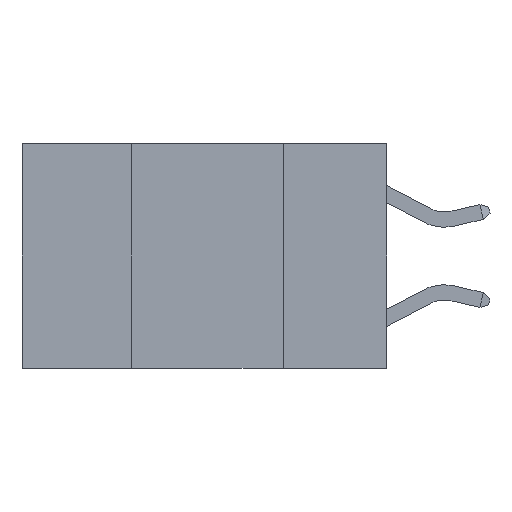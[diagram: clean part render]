
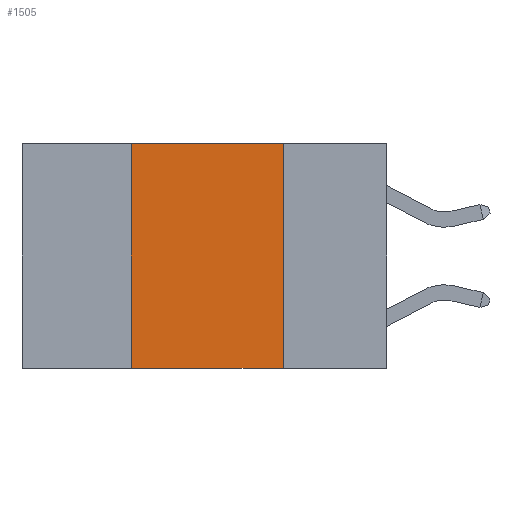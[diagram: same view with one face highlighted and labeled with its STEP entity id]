
A CAD part, left-side view. The second image highlights one B-rep face of the part: STEP entity #1505.
In plain terms, the highlighted planar face has unit normal (-1, 0, 0).
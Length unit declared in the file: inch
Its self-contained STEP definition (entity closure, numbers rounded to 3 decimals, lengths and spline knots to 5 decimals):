
#339 = CARTESIAN_POINT ( 'NONE',  ( 0., 0.17, 0. ) ) ;
#483 = DIRECTION ( 'NONE',  ( 0., 0., 1. ) ) ;
#638 = DIRECTION ( 'NONE',  ( 0., -1., 0. ) ) ;
#950 = CARTESIAN_POINT ( 'NONE',  ( 0., 0.42, 0. ) ) ;
#1000 = VERTEX_POINT ( 'NONE', #4841 ) ;
#1066 = ORIENTED_EDGE ( 'NONE', *, *, #4384, .F. ) ;
#1128 = ORIENTED_EDGE ( 'NONE', *, *, #9726, .F. ) ;
#1137 = ORIENTED_EDGE ( 'NONE', *, *, #7871, .F. ) ;
#1216 = ORIENTED_EDGE ( 'NONE', *, *, #9218, .T. ) ;
#1371 = LINE ( 'NONE', #10041, #9614 ) ;
#1448 = CARTESIAN_POINT ( 'NONE',  ( 0., 0.42, -0.37 ) ) ;
#1505 = ADVANCED_FACE ( 'NONE', ( #4054 ), #2996, .F. ) ;
#1510 = VERTEX_POINT ( 'NONE', #339 ) ;
#1856 = VERTEX_POINT ( 'NONE', #950 ) ;
#2473 = AXIS2_PLACEMENT_3D ( 'NONE', #3830, #4743, #10279 ) ;
#2729 = DIRECTION ( 'NONE',  ( 0., -1., 0. ) ) ;
#2772 = LINE ( 'NONE', #5670, #4814 ) ;
#2848 = EDGE_LOOP ( 'NONE', ( #1066, #1128, #1137, #1216 ) ) ;
#2996 = PLANE ( 'NONE',  #2473 ) ;
#3026 = LINE ( 'NONE', #10499, #7190 ) ;
#3674 = VECTOR ( 'NONE', #8176, 39.37008 ) ;
#3830 = CARTESIAN_POINT ( 'NONE',  ( 0., 0.6, 0. ) ) ;
#4054 = FACE_OUTER_BOUND ( 'NONE', #2848, .T. ) ;
#4384 = EDGE_CURVE ( 'NONE', #1510, #1000, #8034, .T. ) ;
#4743 = DIRECTION ( 'NONE',  ( 1., 0., 0. ) ) ;
#4814 = VECTOR ( 'NONE', #483, 39.37008 ) ;
#4841 = CARTESIAN_POINT ( 'NONE',  ( 0., 0.17, -0.37 ) ) ;
#5670 = CARTESIAN_POINT ( 'NONE',  ( 0., 0.42, 0. ) ) ;
#7190 = VECTOR ( 'NONE', #638, 39.37008 ) ;
#7871 = EDGE_CURVE ( 'NONE', #8722, #1856, #2772, .T. ) ;
#8034 = LINE ( 'NONE', #9678, #3674 ) ;
#8176 = DIRECTION ( 'NONE',  ( 0., 0., -1. ) ) ;
#8722 = VERTEX_POINT ( 'NONE', #1448 ) ;
#9218 = EDGE_CURVE ( 'NONE', #8722, #1000, #1371, .T. ) ;
#9614 = VECTOR ( 'NONE', #2729, 39.37008 ) ;
#9678 = CARTESIAN_POINT ( 'NONE',  ( 0., 0.17, 0. ) ) ;
#9726 = EDGE_CURVE ( 'NONE', #1856, #1510, #3026, .T. ) ;
#10041 = CARTESIAN_POINT ( 'NONE',  ( 0., 0.6, -0.37 ) ) ;
#10279 = DIRECTION ( 'NONE',  ( 0., 0., -1. ) ) ;
#10499 = CARTESIAN_POINT ( 'NONE',  ( 0., 0.6, 0. ) ) ;
